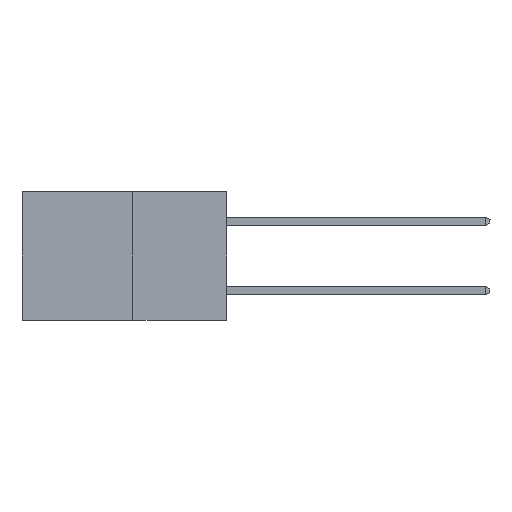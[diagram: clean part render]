
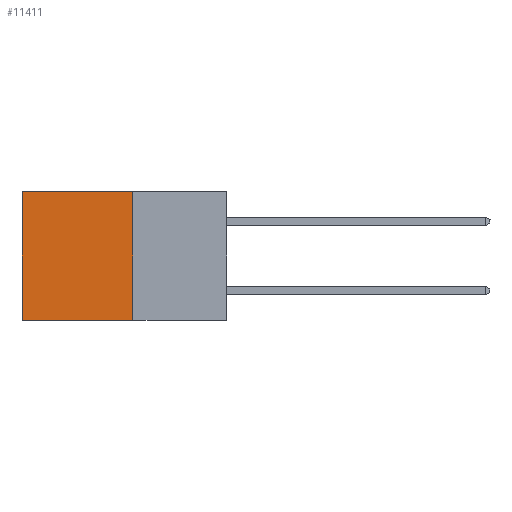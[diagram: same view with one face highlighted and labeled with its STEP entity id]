
A CAD part, left-side view. The second image highlights one B-rep face of the part: STEP entity #11411.
In plain terms, the highlighted planar face has unit normal (-1, 0, 0).
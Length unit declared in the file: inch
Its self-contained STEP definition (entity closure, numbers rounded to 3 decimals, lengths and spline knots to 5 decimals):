
#730 = CARTESIAN_POINT ( 'NONE',  ( 0.277, 0.59, -0.37 ) ) ;
#811 = LINE ( 'NONE', #4914, #6938 ) ;
#1432 = PLANE ( 'NONE',  #14270 ) ;
#2330 = LINE ( 'NONE', #2388, #9149 ) ;
#2388 = CARTESIAN_POINT ( 'NONE',  ( 0.277, 0.59, -0.37 ) ) ;
#2662 = CARTESIAN_POINT ( 'NONE',  ( 0.277, 0.27, -0.37 ) ) ;
#2737 = EDGE_CURVE ( 'NONE', #13601, #13737, #5387, .T. ) ;
#3347 = EDGE_LOOP ( 'NONE', ( #9717, #5563, #13118, #14614 ) ) ;
#3899 = DIRECTION ( 'NONE',  ( 1., 0., 0. ) ) ;
#4108 = EDGE_CURVE ( 'NONE', #13737, #10361, #2330, .T. ) ;
#4646 = VECTOR ( 'NONE', #8099, 39.37008 ) ;
#4914 = CARTESIAN_POINT ( 'NONE',  ( 0.277, 0.27, -0.37 ) ) ;
#5387 = LINE ( 'NONE', #13135, #11046 ) ;
#5563 = ORIENTED_EDGE ( 'NONE', *, *, #13400, .F. ) ;
#6117 = CARTESIAN_POINT ( 'NONE',  ( 0.277, 0.27, -0.37 ) ) ;
#6125 = EDGE_CURVE ( 'NONE', #13601, #6261, #11055, .T. ) ;
#6140 = DIRECTION ( 'NONE',  ( 0., 1., 0. ) ) ;
#6261 = VERTEX_POINT ( 'NONE', #6117 ) ;
#6938 = VECTOR ( 'NONE', #6140, 39.37008 ) ;
#7473 = DIRECTION ( 'NONE',  ( 0., 0., -1. ) ) ;
#8097 = CARTESIAN_POINT ( 'NONE',  ( 0.277, 0.27, -0.37 ) ) ;
#8099 = DIRECTION ( 'NONE',  ( 0., 0., -1. ) ) ;
#8875 = CARTESIAN_POINT ( 'NONE',  ( 0.277, 0.27, 0. ) ) ;
#9149 = VECTOR ( 'NONE', #7473, 39.37008 ) ;
#9717 = ORIENTED_EDGE ( 'NONE', *, *, #4108, .T. ) ;
#10361 = VERTEX_POINT ( 'NONE', #730 ) ;
#11046 = VECTOR ( 'NONE', #12919, 39.37008 ) ;
#11055 = LINE ( 'NONE', #8097, #4646 ) ;
#11411 = ADVANCED_FACE ( 'NONE', ( #14656 ), #1432, .F. ) ;
#12323 = DIRECTION ( 'NONE',  ( 0., 0., -1. ) ) ;
#12919 = DIRECTION ( 'NONE',  ( 0., 1., 0. ) ) ;
#13118 = ORIENTED_EDGE ( 'NONE', *, *, #6125, .F. ) ;
#13135 = CARTESIAN_POINT ( 'NONE',  ( 0.277, 0.27, 0. ) ) ;
#13400 = EDGE_CURVE ( 'NONE', #6261, #10361, #811, .T. ) ;
#13601 = VERTEX_POINT ( 'NONE', #8875 ) ;
#13737 = VERTEX_POINT ( 'NONE', #13965 ) ;
#13965 = CARTESIAN_POINT ( 'NONE',  ( 0.277, 0.59, 0. ) ) ;
#14270 = AXIS2_PLACEMENT_3D ( 'NONE', #2662, #3899, #12323 ) ;
#14614 = ORIENTED_EDGE ( 'NONE', *, *, #2737, .T. ) ;
#14656 = FACE_OUTER_BOUND ( 'NONE', #3347, .T. ) ;
